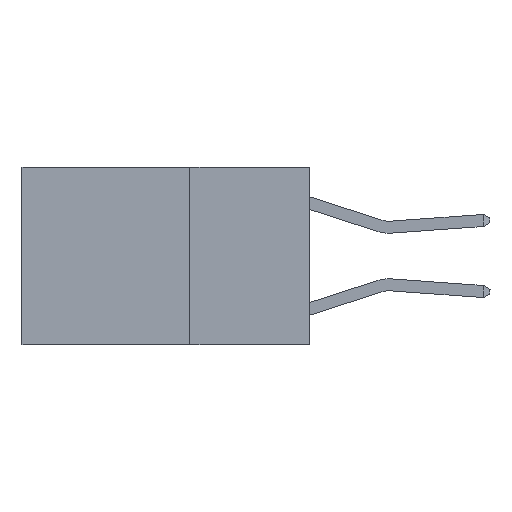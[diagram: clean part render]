
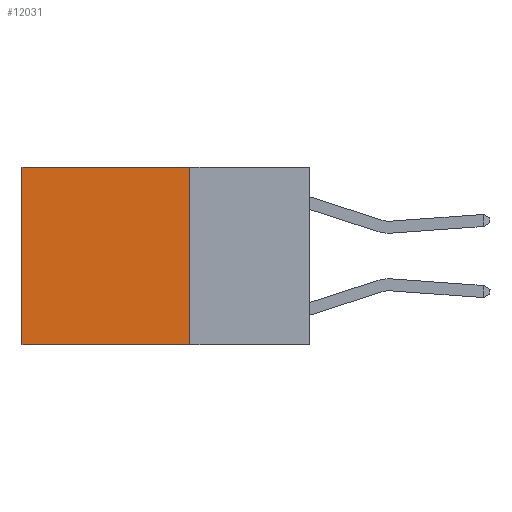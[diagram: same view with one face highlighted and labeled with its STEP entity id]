
A CAD part, left-side view. The second image highlights one B-rep face of the part: STEP entity #12031.
In plain terms, the highlighted planar face has unit normal (-1, 0, 0).
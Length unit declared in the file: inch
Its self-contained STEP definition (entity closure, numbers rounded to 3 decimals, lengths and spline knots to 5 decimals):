
#187 = VERTEX_POINT ( 'NONE', #7062 ) ;
#359 = CARTESIAN_POINT ( 'NONE',  ( 0.2625, 0.6, 0. ) ) ;
#448 = VECTOR ( 'NONE', #14965, 39.37008 ) ;
#639 = VERTEX_POINT ( 'NONE', #5536 ) ;
#853 = ORIENTED_EDGE ( 'NONE', *, *, #3313, .F. ) ;
#1356 = CARTESIAN_POINT ( 'NONE',  ( 0.2625, 0.25, -0.37 ) ) ;
#1898 = AXIS2_PLACEMENT_3D ( 'NONE', #6139, #6491, #10328 ) ;
#2180 = CARTESIAN_POINT ( 'NONE',  ( 0.2625, 0.25, 0. ) ) ;
#2522 = LINE ( 'NONE', #9135, #8374 ) ;
#3313 = EDGE_CURVE ( 'NONE', #5018, #187, #3324, .T. ) ;
#3324 = LINE ( 'NONE', #11189, #16583 ) ;
#3331 = EDGE_LOOP ( 'NONE', ( #11178, #12489, #853, #9730 ) ) ;
#4769 = VECTOR ( 'NONE', #6380, 39.37008 ) ;
#5018 = VERTEX_POINT ( 'NONE', #2180 ) ;
#5536 = CARTESIAN_POINT ( 'NONE',  ( 0.2625, 0.6, -0.37 ) ) ;
#6139 = CARTESIAN_POINT ( 'NONE',  ( 0.2625, 0.25, 0. ) ) ;
#6380 = DIRECTION ( 'NONE',  ( 0., 1., 0. ) ) ;
#6491 = DIRECTION ( 'NONE',  ( 1., 0., 0. ) ) ;
#7062 = CARTESIAN_POINT ( 'NONE',  ( 0.2625, 0.25, -0.37 ) ) ;
#7568 = PLANE ( 'NONE',  #1898 ) ;
#7634 = CARTESIAN_POINT ( 'NONE',  ( 0.2625, 0.25, 0. ) ) ;
#7824 = FACE_OUTER_BOUND ( 'NONE', #3331, .T. ) ;
#8374 = VECTOR ( 'NONE', #9051, 39.37008 ) ;
#8572 = EDGE_CURVE ( 'NONE', #187, #639, #14610, .T. ) ;
#9051 = DIRECTION ( 'NONE',  ( 0., 0., -1. ) ) ;
#9135 = CARTESIAN_POINT ( 'NONE',  ( 0.2625, 0.6, 0. ) ) ;
#9305 = EDGE_CURVE ( 'NONE', #13348, #639, #2522, .T. ) ;
#9730 = ORIENTED_EDGE ( 'NONE', *, *, #14193, .T. ) ;
#10328 = DIRECTION ( 'NONE',  ( 0., 0., -1. ) ) ;
#11178 = ORIENTED_EDGE ( 'NONE', *, *, #9305, .T. ) ;
#11189 = CARTESIAN_POINT ( 'NONE',  ( 0.2625, 0.25, 0. ) ) ;
#11277 = DIRECTION ( 'NONE',  ( 0., 0., -1. ) ) ;
#12031 = ADVANCED_FACE ( 'NONE', ( #7824 ), #7568, .F. ) ;
#12489 = ORIENTED_EDGE ( 'NONE', *, *, #8572, .F. ) ;
#13181 = LINE ( 'NONE', #7634, #4769 ) ;
#13348 = VERTEX_POINT ( 'NONE', #359 ) ;
#14193 = EDGE_CURVE ( 'NONE', #5018, #13348, #13181, .T. ) ;
#14610 = LINE ( 'NONE', #1356, #448 ) ;
#14965 = DIRECTION ( 'NONE',  ( 0., 1., 0. ) ) ;
#16583 = VECTOR ( 'NONE', #11277, 39.37008 ) ;
